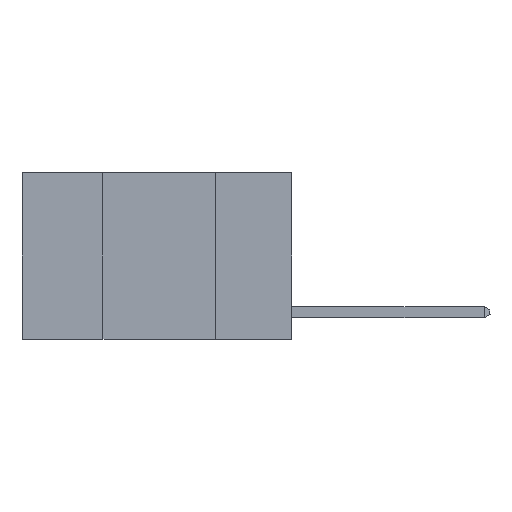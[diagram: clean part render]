
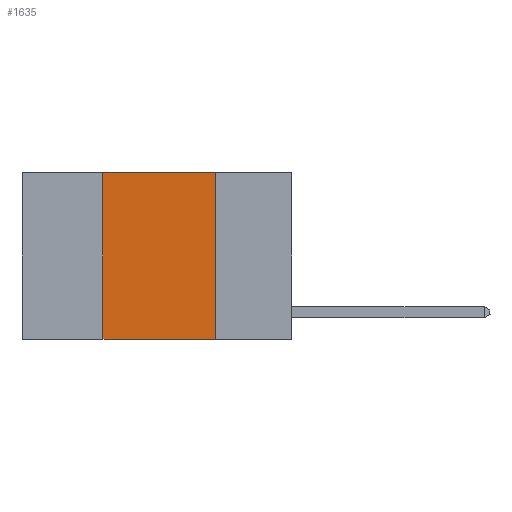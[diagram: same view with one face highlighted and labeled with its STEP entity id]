
A CAD part, left-side view. The second image highlights one B-rep face of the part: STEP entity #1635.
In plain terms, the highlighted planar face has unit normal (-1, 0, 0).
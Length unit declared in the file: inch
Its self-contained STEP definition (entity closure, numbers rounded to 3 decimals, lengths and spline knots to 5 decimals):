
#36 = CARTESIAN_POINT ( 'NONE',  ( 0., 0.17, 0. ) ) ;
#332 = DIRECTION ( 'NONE',  ( 1., 0., 0. ) ) ;
#1207 = EDGE_CURVE ( 'NONE', #18640, #3914, #4699, .T. ) ;
#1635 = ADVANCED_FACE ( 'NONE', ( #23783 ), #4550, .F. ) ;
#2704 = AXIS2_PLACEMENT_3D ( 'NONE', #17799, #332, #16124 ) ;
#2814 = EDGE_CURVE ( 'NONE', #9231, #8517, #13603, .T. ) ;
#3914 = VERTEX_POINT ( 'NONE', #14462 ) ;
#4320 = VECTOR ( 'NONE', #21964, 39.37008 ) ;
#4550 = PLANE ( 'NONE',  #2704 ) ;
#4699 = LINE ( 'NONE', #6731, #9581 ) ;
#6045 = CARTESIAN_POINT ( 'NONE',  ( 0., 0.42, 0. ) ) ;
#6731 = CARTESIAN_POINT ( 'NONE',  ( 0., 0.6, -0.37 ) ) ;
#7117 = ORIENTED_EDGE ( 'NONE', *, *, #1207, .T. ) ;
#7889 = DIRECTION ( 'NONE',  ( 0., -1., 0. ) ) ;
#8310 = CARTESIAN_POINT ( 'NONE',  ( 0., 0.42, 0. ) ) ;
#8376 = CARTESIAN_POINT ( 'NONE',  ( 0., 0.42, -0.37 ) ) ;
#8517 = VERTEX_POINT ( 'NONE', #36 ) ;
#9231 = VERTEX_POINT ( 'NONE', #8310 ) ;
#9581 = VECTOR ( 'NONE', #18200, 39.37008 ) ;
#12625 = ORIENTED_EDGE ( 'NONE', *, *, #2814, .F. ) ;
#13099 = VECTOR ( 'NONE', #7889, 39.37008 ) ;
#13485 = ORIENTED_EDGE ( 'NONE', *, *, #21610, .F. ) ;
#13603 = LINE ( 'NONE', #23540, #13099 ) ;
#14462 = CARTESIAN_POINT ( 'NONE',  ( 0., 0.17, -0.37 ) ) ;
#15645 = EDGE_LOOP ( 'NONE', ( #25008, #12625, #13485, #7117 ) ) ;
#16124 = DIRECTION ( 'NONE',  ( 0., 0., -1. ) ) ;
#17799 = CARTESIAN_POINT ( 'NONE',  ( 0., 0.6, 0. ) ) ;
#18200 = DIRECTION ( 'NONE',  ( 0., -1., 0. ) ) ;
#18640 = VERTEX_POINT ( 'NONE', #8376 ) ;
#19675 = LINE ( 'NONE', #6045, #20875 ) ;
#20875 = VECTOR ( 'NONE', #21337, 39.37008 ) ;
#21337 = DIRECTION ( 'NONE',  ( 0., 0., 1. ) ) ;
#21596 = CARTESIAN_POINT ( 'NONE',  ( 0., 0.17, 0. ) ) ;
#21610 = EDGE_CURVE ( 'NONE', #18640, #9231, #19675, .T. ) ;
#21964 = DIRECTION ( 'NONE',  ( 0., 0., -1. ) ) ;
#23540 = CARTESIAN_POINT ( 'NONE',  ( 0., 0.6, 0. ) ) ;
#23783 = FACE_OUTER_BOUND ( 'NONE', #15645, .T. ) ;
#23871 = LINE ( 'NONE', #21596, #4320 ) ;
#24537 = EDGE_CURVE ( 'NONE', #8517, #3914, #23871, .T. ) ;
#25008 = ORIENTED_EDGE ( 'NONE', *, *, #24537, .F. ) ;
